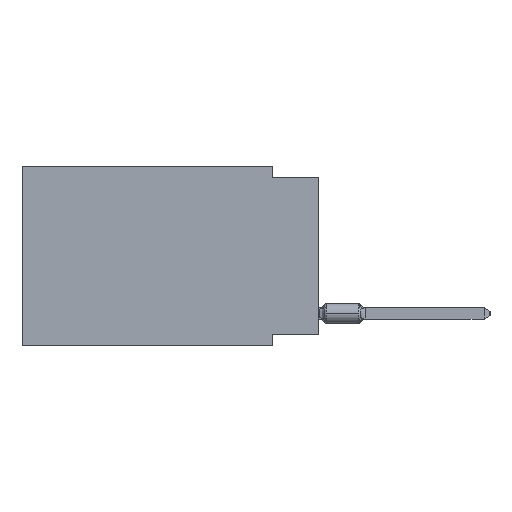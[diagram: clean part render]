
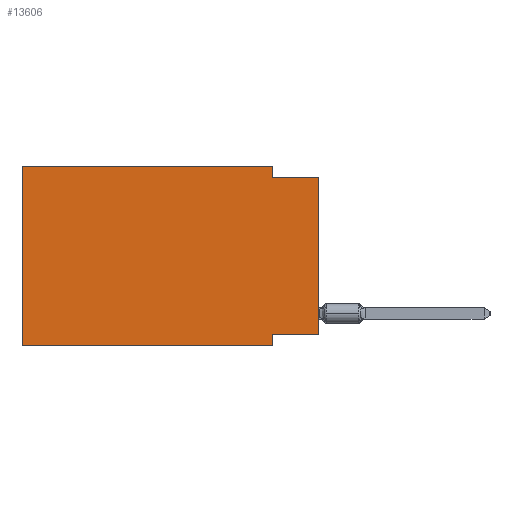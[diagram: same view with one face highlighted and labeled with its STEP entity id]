
A CAD part, left-side view. The second image highlights one B-rep face of the part: STEP entity #13606.
In plain terms, the highlighted planar face has unit normal (-1, 0, 0).
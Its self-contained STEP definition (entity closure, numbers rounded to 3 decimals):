
#1130 = DIRECTION ( 'NONE',  ( 0., 0., -1. ) ) ;
#4903 = LINE ( 'NONE', #28294, #9731 ) ;
#5125 = VERTEX_POINT ( 'NONE', #65623 ) ;
#6063 = CARTESIAN_POINT ( 'NONE',  ( 0., 0., 0. ) ) ;
#9731 = VECTOR ( 'NONE', #22542, 1000. ) ;
#11339 = FACE_OUTER_BOUND ( 'NONE', #37338, .T. ) ;
#11560 = ORIENTED_EDGE ( 'NONE', *, *, #51879, .T. ) ;
#11716 = CARTESIAN_POINT ( 'NONE',  ( 0., 16.383, 0. ) ) ;
#12115 = EDGE_CURVE ( 'NONE', #28747, #22975, #4903, .T. ) ;
#12657 = VERTEX_POINT ( 'NONE', #31586 ) ;
#13606 = ADVANCED_FACE ( 'NONE', ( #11339 ), #64211, .F. ) ;
#15130 = VERTEX_POINT ( 'NONE', #29672 ) ;
#16981 = DIRECTION ( 'NONE',  ( 0., -1., 0. ) ) ;
#17495 = VECTOR ( 'NONE', #16981, 1000. ) ;
#17736 = LINE ( 'NONE', #41086, #17495 ) ;
#18963 = LINE ( 'NONE', #35840, #52781 ) ;
#19072 = LINE ( 'NONE', #6063, #50162 ) ;
#19680 = EDGE_CURVE ( 'NONE', #60278, #15130, #60898, .T. ) ;
#19908 = EDGE_CURVE ( 'NONE', #22975, #60278, #35179, .T. ) ;
#21990 = AXIS2_PLACEMENT_3D ( 'NONE', #11716, #34719, #63070 ) ;
#22542 = DIRECTION ( 'NONE',  ( 0., 0., 1. ) ) ;
#22948 = EDGE_CURVE ( 'NONE', #15130, #24121, #17736, .T. ) ;
#22975 = VERTEX_POINT ( 'NONE', #36102 ) ;
#23083 = CARTESIAN_POINT ( 'NONE',  ( 0., 0., -9.271 ) ) ;
#24048 = DIRECTION ( 'NONE',  ( 0., -1., 0. ) ) ;
#24121 = VERTEX_POINT ( 'NONE', #33570 ) ;
#24441 = CARTESIAN_POINT ( 'NONE',  ( 0., 2.54, -9.906 ) ) ;
#26550 = ORIENTED_EDGE ( 'NONE', *, *, #22948, .F. ) ;
#27281 = VECTOR ( 'NONE', #1130, 1000. ) ;
#28294 = CARTESIAN_POINT ( 'NONE',  ( 0., 16.383, 0. ) ) ;
#28747 = VERTEX_POINT ( 'NONE', #60324 ) ;
#29174 = ORIENTED_EDGE ( 'NONE', *, *, #19908, .F. ) ;
#29204 = DIRECTION ( 'NONE',  ( 0., 1., 0. ) ) ;
#29672 = CARTESIAN_POINT ( 'NONE',  ( 0., 2.54, -0.635 ) ) ;
#31586 = CARTESIAN_POINT ( 'NONE',  ( 0., 0., -9.271 ) ) ;
#31830 = VECTOR ( 'NONE', #65054, 1000. ) ;
#33570 = CARTESIAN_POINT ( 'NONE',  ( 0., 0., -0.635 ) ) ;
#34353 = ORIENTED_EDGE ( 'NONE', *, *, #53925, .F. ) ;
#34719 = DIRECTION ( 'NONE',  ( 1., 0., 0. ) ) ;
#35179 = LINE ( 'NONE', #40551, #65279 ) ;
#35840 = CARTESIAN_POINT ( 'NONE',  ( 0., 16.383, -9.906 ) ) ;
#36102 = CARTESIAN_POINT ( 'NONE',  ( 0., 16.383, 0. ) ) ;
#37338 = EDGE_LOOP ( 'NONE', ( #11560, #26550, #63786, #29174, #44734, #55846, #34353, #61053 ) ) ;
#40551 = CARTESIAN_POINT ( 'NONE',  ( 0., 16.383, 0. ) ) ;
#41086 = CARTESIAN_POINT ( 'NONE',  ( 0., 0., -0.635 ) ) ;
#42325 = DIRECTION ( 'NONE',  ( 0., -1., 0. ) ) ;
#42429 = DIRECTION ( 'NONE',  ( 0., 0., 1. ) ) ;
#44734 = ORIENTED_EDGE ( 'NONE', *, *, #12115, .F. ) ;
#47884 = CARTESIAN_POINT ( 'NONE',  ( 0., 2.54, 0. ) ) ;
#48514 = EDGE_CURVE ( 'NONE', #28747, #5125, #18963, .T. ) ;
#50162 = VECTOR ( 'NONE', #42429, 1000. ) ;
#51879 = EDGE_CURVE ( 'NONE', #12657, #24121, #19072, .T. ) ;
#52687 = CARTESIAN_POINT ( 'NONE',  ( 0., 2.54, 0. ) ) ;
#52781 = VECTOR ( 'NONE', #42325, 1000. ) ;
#52953 = LINE ( 'NONE', #23083, #66845 ) ;
#53541 = LINE ( 'NONE', #24441, #31830 ) ;
#53925 = EDGE_CURVE ( 'NONE', #64474, #5125, #53541, .T. ) ;
#55846 = ORIENTED_EDGE ( 'NONE', *, *, #48514, .T. ) ;
#60278 = VERTEX_POINT ( 'NONE', #52687 ) ;
#60324 = CARTESIAN_POINT ( 'NONE',  ( 0., 16.383, -9.906 ) ) ;
#60898 = LINE ( 'NONE', #47884, #27281 ) ;
#61053 = ORIENTED_EDGE ( 'NONE', *, *, #68944, .F. ) ;
#63070 = DIRECTION ( 'NONE',  ( 0., 0., -1. ) ) ;
#63786 = ORIENTED_EDGE ( 'NONE', *, *, #19680, .F. ) ;
#64211 = PLANE ( 'NONE',  #21990 ) ;
#64474 = VERTEX_POINT ( 'NONE', #73728 ) ;
#65054 = DIRECTION ( 'NONE',  ( 0., 0., -1. ) ) ;
#65279 = VECTOR ( 'NONE', #24048, 1000. ) ;
#65623 = CARTESIAN_POINT ( 'NONE',  ( 0., 2.54, -9.906 ) ) ;
#66845 = VECTOR ( 'NONE', #29204, 1000. ) ;
#68944 = EDGE_CURVE ( 'NONE', #12657, #64474, #52953, .T. ) ;
#73728 = CARTESIAN_POINT ( 'NONE',  ( 0., 2.54, -9.271 ) ) ;
